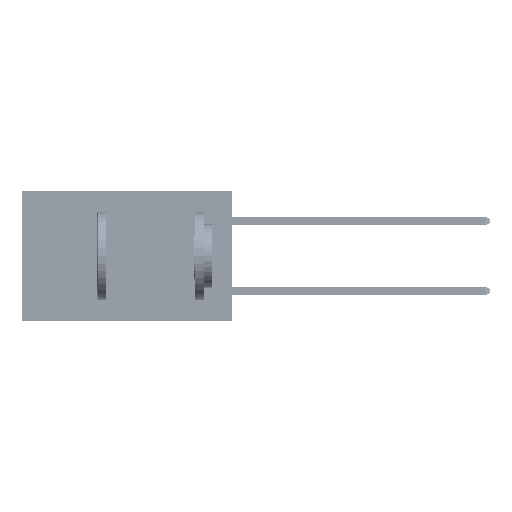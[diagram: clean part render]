
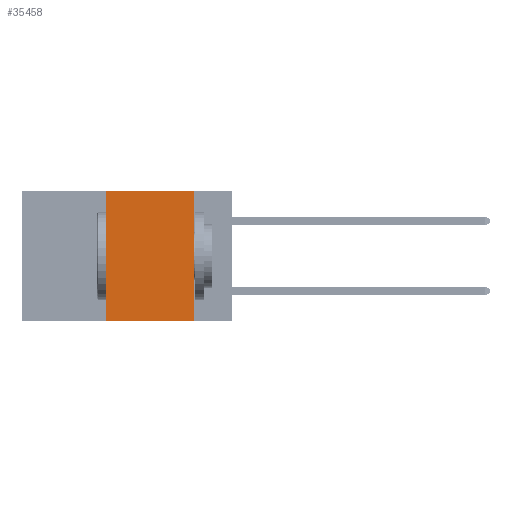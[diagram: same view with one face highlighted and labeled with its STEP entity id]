
A CAD part, left-side view. The second image highlights one B-rep face of the part: STEP entity #35458.
In plain terms, the highlighted planar face has unit normal (-1, 0, 0).
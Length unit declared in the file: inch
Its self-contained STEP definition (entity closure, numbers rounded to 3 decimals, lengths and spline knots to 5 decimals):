
#2894 = VECTOR ( 'NONE', #4099, 39.37008 ) ;
#4099 = DIRECTION ( 'NONE',  ( 0., 0., 1. ) ) ;
#4331 = PLANE ( 'NONE',  #5953 ) ;
#4648 = CARTESIAN_POINT ( 'NONE',  ( 0., 0.36, -0.37 ) ) ;
#5091 = EDGE_CURVE ( 'NONE', #30645, #50567, #22356, .T. ) ;
#5953 = AXIS2_PLACEMENT_3D ( 'NONE', #41387, #16871, #45483 ) ;
#8762 = CARTESIAN_POINT ( 'NONE',  ( 0., 0.36, 0. ) ) ;
#8848 = DIRECTION ( 'NONE',  ( 0., 0., -1. ) ) ;
#10542 = VERTEX_POINT ( 'NONE', #47861 ) ;
#12792 = FACE_OUTER_BOUND ( 'NONE', #51968, .T. ) ;
#13879 = VERTEX_POINT ( 'NONE', #14956 ) ;
#14956 = CARTESIAN_POINT ( 'NONE',  ( 0., 0.11, -0.37 ) ) ;
#16746 = LINE ( 'NONE', #53100, #26362 ) ;
#16871 = DIRECTION ( 'NONE',  ( 1., 0., 0. ) ) ;
#22356 = LINE ( 'NONE', #32939, #2894 ) ;
#24215 = EDGE_CURVE ( 'NONE', #10542, #13879, #51827, .T. ) ;
#25316 = DIRECTION ( 'NONE',  ( 0., -1., 0. ) ) ;
#26362 = VECTOR ( 'NONE', #45131, 39.37008 ) ;
#29392 = CARTESIAN_POINT ( 'NONE',  ( 0., 0.11, 0. ) ) ;
#30645 = VERTEX_POINT ( 'NONE', #4648 ) ;
#32939 = CARTESIAN_POINT ( 'NONE',  ( 0., 0.36, 0. ) ) ;
#35392 = EDGE_CURVE ( 'NONE', #30645, #13879, #16746, .T. ) ;
#35458 = ADVANCED_FACE ( 'NONE', ( #12792 ), #4331, .F. ) ;
#38782 = ORIENTED_EDGE ( 'NONE', *, *, #40095, .F. ) ;
#39902 = LINE ( 'NONE', #41587, #49447 ) ;
#40030 = ORIENTED_EDGE ( 'NONE', *, *, #5091, .F. ) ;
#40095 = EDGE_CURVE ( 'NONE', #50567, #10542, #39902, .T. ) ;
#41387 = CARTESIAN_POINT ( 'NONE',  ( 0., 0.6, 0. ) ) ;
#41587 = CARTESIAN_POINT ( 'NONE',  ( 0., 0.6, 0. ) ) ;
#42307 = VECTOR ( 'NONE', #8848, 39.37008 ) ;
#44488 = ORIENTED_EDGE ( 'NONE', *, *, #24215, .F. ) ;
#45131 = DIRECTION ( 'NONE',  ( 0., -1., 0. ) ) ;
#45193 = ORIENTED_EDGE ( 'NONE', *, *, #35392, .T. ) ;
#45483 = DIRECTION ( 'NONE',  ( 0., 0., -1. ) ) ;
#47861 = CARTESIAN_POINT ( 'NONE',  ( 0., 0.11, 0. ) ) ;
#49447 = VECTOR ( 'NONE', #25316, 39.37008 ) ;
#50567 = VERTEX_POINT ( 'NONE', #8762 ) ;
#51827 = LINE ( 'NONE', #29392, #42307 ) ;
#51968 = EDGE_LOOP ( 'NONE', ( #44488, #38782, #40030, #45193 ) ) ;
#53100 = CARTESIAN_POINT ( 'NONE',  ( 0., 0.6, -0.37 ) ) ;
